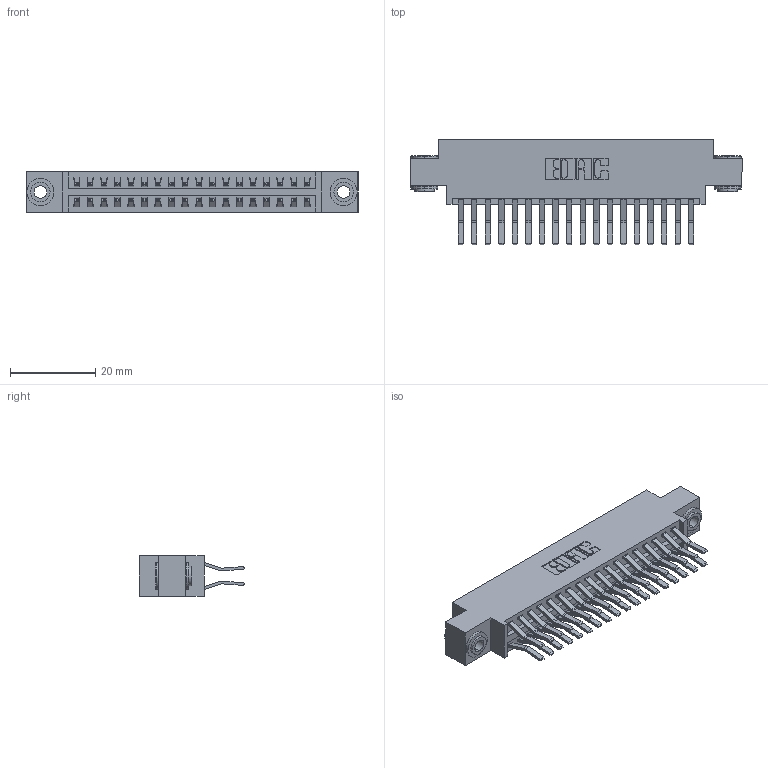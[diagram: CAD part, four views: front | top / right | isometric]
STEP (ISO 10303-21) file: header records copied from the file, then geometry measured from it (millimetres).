
FILE_DESCRIPTION (( 'STEP AP203' ), '1' );
FILE_NAME ('396-036-560-803.STEP', '2019-11-02T05:19:39', ( '' ), ( '' ), 'SwSTEP 2.0', 'SolidWorks 2016', '' );
FILE_SCHEMA (( 'CONFIG_CONTROL_DESIGN' ));
Length unit declared in the file: inch
Products named in the file (4): 396-036-560-803; 346 Part_0.170 Offset - 0.156 Dia-TH; 345-292-001_560 Tail; 345-250-002_345-250-002-102
Assembly tree (39 placements, depth 2):
  396-036-560-803
    346 Part_0.170 Offset - 0.156 Dia-TH
    345-292-001_560 Tail  x36
    345-250-002_345-250-002-102  x2
Bounding box: 77.72 x 24.78 x 9.4 mm (x, y, z)
Volume: 7493.4 mm3; surface area: 10946.3 mm2
Topology: 39 solids, 39 shells, 2108 faces, 6213 edges, 4090 vertices
Faces by surface type: plane 1350, cylinder 750, cone 8
Entity records: 15848 total; most frequent: CARTESIAN_POINT 2623, ORIENTED_EDGE 2550, DIRECTION 2397, EDGE_CURVE 1275, VECTOR 1043, LINE 1043, VERTEX_POINT 846, AXIS2_PLACEMENT_3D 677
